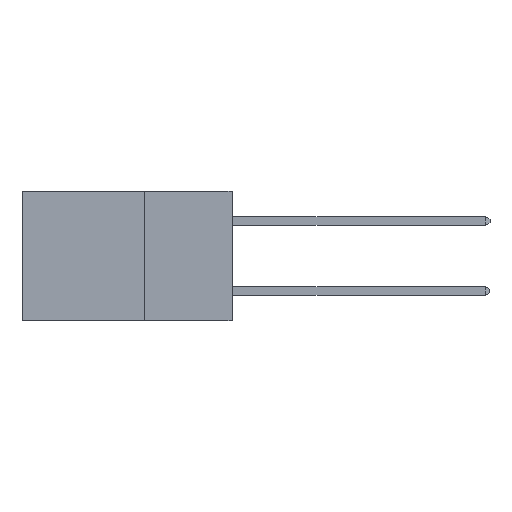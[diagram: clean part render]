
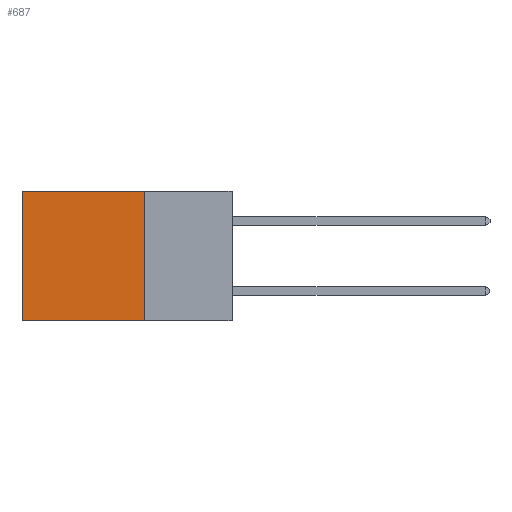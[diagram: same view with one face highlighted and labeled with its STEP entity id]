
A CAD part, left-side view. The second image highlights one B-rep face of the part: STEP entity #687.
In plain terms, the highlighted planar face has unit normal (-1, 0, 0).
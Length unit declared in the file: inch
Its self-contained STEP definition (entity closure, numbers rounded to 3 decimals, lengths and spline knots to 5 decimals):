
#38 = VERTEX_POINT ( 'NONE', #11277 ) ;
#687 = ADVANCED_FACE ( 'NONE', ( #10665 ), #7594, .F. ) ;
#1418 = VECTOR ( 'NONE', #14896, 39.37008 ) ;
#1900 = CARTESIAN_POINT ( 'NONE',  ( 0.2875, 0.25, 0. ) ) ;
#2409 = VERTEX_POINT ( 'NONE', #23182 ) ;
#3197 = VECTOR ( 'NONE', #21920, 39.37008 ) ;
#3971 = EDGE_CURVE ( 'NONE', #38, #17338, #16586, .T. ) ;
#4134 = CARTESIAN_POINT ( 'NONE',  ( 0.2875, 0.25, 0. ) ) ;
#5650 = DIRECTION ( 'NONE',  ( 0., 1., 0. ) ) ;
#5880 = CARTESIAN_POINT ( 'NONE',  ( 0.2875, 0.6, 0. ) ) ;
#6056 = VECTOR ( 'NONE', #5650, 39.37008 ) ;
#6269 = ORIENTED_EDGE ( 'NONE', *, *, #11007, .T. ) ;
#6364 = VECTOR ( 'NONE', #16853, 39.37008 ) ;
#6467 = LINE ( 'NONE', #11257, #1418 ) ;
#7052 = DIRECTION ( 'NONE',  ( 0., 0., -1. ) ) ;
#7542 = DIRECTION ( 'NONE',  ( 1., 0., 0. ) ) ;
#7594 = PLANE ( 'NONE',  #15604 ) ;
#7894 = EDGE_CURVE ( 'NONE', #18196, #2409, #13595, .T. ) ;
#8470 = CARTESIAN_POINT ( 'NONE',  ( 0.2875, 0.6, -0.37 ) ) ;
#10665 = FACE_OUTER_BOUND ( 'NONE', #20441, .T. ) ;
#11007 = EDGE_CURVE ( 'NONE', #18196, #38, #6467, .T. ) ;
#11257 = CARTESIAN_POINT ( 'NONE',  ( 0.2875, 0.25, 0. ) ) ;
#11277 = CARTESIAN_POINT ( 'NONE',  ( 0.2875, 0.6, 0. ) ) ;
#12861 = ORIENTED_EDGE ( 'NONE', *, *, #7894, .F. ) ;
#12972 = ORIENTED_EDGE ( 'NONE', *, *, #3971, .T. ) ;
#13069 = CARTESIAN_POINT ( 'NONE',  ( 0.2875, 0.25, 0. ) ) ;
#13497 = EDGE_CURVE ( 'NONE', #2409, #17338, #15732, .T. ) ;
#13595 = LINE ( 'NONE', #1900, #3197 ) ;
#14896 = DIRECTION ( 'NONE',  ( 0., 1., 0. ) ) ;
#15604 = AXIS2_PLACEMENT_3D ( 'NONE', #4134, #7542, #7052 ) ;
#15732 = LINE ( 'NONE', #21912, #6056 ) ;
#16586 = LINE ( 'NONE', #5880, #6364 ) ;
#16853 = DIRECTION ( 'NONE',  ( 0., 0., -1. ) ) ;
#17338 = VERTEX_POINT ( 'NONE', #8470 ) ;
#18196 = VERTEX_POINT ( 'NONE', #13069 ) ;
#20441 = EDGE_LOOP ( 'NONE', ( #12972, #22972, #12861, #6269 ) ) ;
#21912 = CARTESIAN_POINT ( 'NONE',  ( 0.2875, 0.25, -0.37 ) ) ;
#21920 = DIRECTION ( 'NONE',  ( 0., 0., -1. ) ) ;
#22972 = ORIENTED_EDGE ( 'NONE', *, *, #13497, .F. ) ;
#23182 = CARTESIAN_POINT ( 'NONE',  ( 0.2875, 0.25, -0.37 ) ) ;
